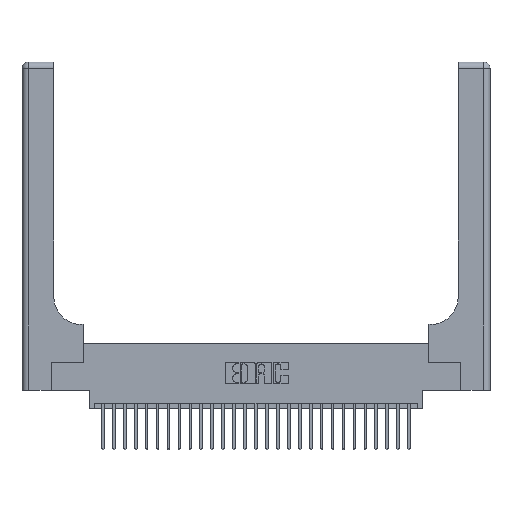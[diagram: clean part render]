
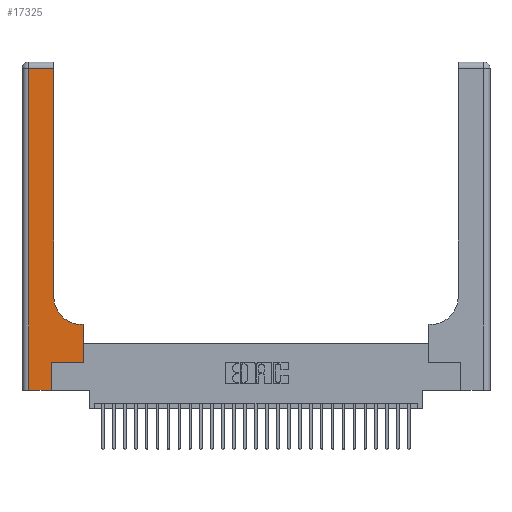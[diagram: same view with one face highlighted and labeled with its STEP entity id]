
A CAD part, top view. The second image highlights one B-rep face of the part: STEP entity #17325.
In plain terms, the highlighted planar face has unit normal (0, 0, 1).
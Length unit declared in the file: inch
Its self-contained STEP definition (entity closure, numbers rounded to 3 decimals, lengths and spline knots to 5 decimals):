
#1298 = LINE ( 'NONE', #27230, #19099 ) ;
#1423 = CARTESIAN_POINT ( 'NONE',  ( 0., 0., 0.37 ) ) ;
#1466 = EDGE_CURVE ( 'NONE', #2934, #4281, #10617, .T. ) ;
#1801 = LINE ( 'NONE', #24195, #18869 ) ;
#2200 = DIRECTION ( 'NONE',  ( 0., 0., -1. ) ) ;
#2375 = CARTESIAN_POINT ( 'NONE',  ( 0.06, 0., 0.37 ) ) ;
#2383 = LINE ( 'NONE', #25163, #8581 ) ;
#2589 = CARTESIAN_POINT ( 'NONE',  ( 0.2915, 0.85, 0.37 ) ) ;
#2788 = ORIENTED_EDGE ( 'NONE', *, *, #9597, .T. ) ;
#2934 = VERTEX_POINT ( 'NONE', #28388 ) ;
#4281 = VERTEX_POINT ( 'NONE', #19247 ) ;
#4468 = DIRECTION ( 'NONE',  ( 0., 1., 0. ) ) ;
#4503 = ORIENTED_EDGE ( 'NONE', *, *, #10538, .T. ) ;
#5629 = ORIENTED_EDGE ( 'NONE', *, *, #15388, .T. ) ;
#5668 = DIRECTION ( 'NONE',  ( 0., -1., 0. ) ) ;
#6126 = VECTOR ( 'NONE', #29009, 39.37008 ) ;
#6192 = CARTESIAN_POINT ( 'NONE',  ( 0.06, 3., 0.37 ) ) ;
#7147 = VERTEX_POINT ( 'NONE', #21695 ) ;
#7614 = ORIENTED_EDGE ( 'NONE', *, *, #24966, .T. ) ;
#8573 = ORIENTED_EDGE ( 'NONE', *, *, #11601, .T. ) ;
#8581 = VECTOR ( 'NONE', #8957, 39.37008 ) ;
#8632 = AXIS2_PLACEMENT_3D ( 'NONE', #16107, #2200, #18460 ) ;
#8703 = CARTESIAN_POINT ( 'NONE',  ( 0.269, 0., 0.37 ) ) ;
#8957 = DIRECTION ( 'NONE',  ( 0., 1., 0. ) ) ;
#9030 = CARTESIAN_POINT ( 'NONE',  ( 0.5585, 0.25, 0.37 ) ) ;
#9222 = VERTEX_POINT ( 'NONE', #16015 ) ;
#9597 = EDGE_CURVE ( 'NONE', #4281, #28077, #13017, .T. ) ;
#10387 = CARTESIAN_POINT ( 'NONE',  ( 0.269, 0.25, 0.37 ) ) ;
#10538 = EDGE_CURVE ( 'NONE', #27369, #9222, #2383, .T. ) ;
#10617 = LINE ( 'NONE', #9030, #22215 ) ;
#11234 = CARTESIAN_POINT ( 'NONE',  ( 0., 3., 0.37 ) ) ;
#11256 = EDGE_CURVE ( 'NONE', #28077, #27369, #25201, .T. ) ;
#11601 = EDGE_CURVE ( 'NONE', #17575, #12013, #23376, .T. ) ;
#12013 = VERTEX_POINT ( 'NONE', #2375 ) ;
#12656 = DIRECTION ( 'NONE',  ( 1., 0., 0. ) ) ;
#13004 = EDGE_CURVE ( 'NONE', #12013, #7147, #28109, .T. ) ;
#13017 = LINE ( 'NONE', #22186, #6126 ) ;
#13105 = DIRECTION ( 'NONE',  ( 1., 0., 0. ) ) ;
#13462 = ORIENTED_EDGE ( 'NONE', *, *, #11256, .T. ) ;
#13506 = CARTESIAN_POINT ( 'NONE',  ( 0.06, 2.94, 0.37 ) ) ;
#13559 = DIRECTION ( 'NONE',  ( 0., 0., -1. ) ) ;
#14509 = ORIENTED_EDGE ( 'NONE', *, *, #29144, .T. ) ;
#15388 = EDGE_CURVE ( 'NONE', #7147, #29729, #26289, .T. ) ;
#15989 = VECTOR ( 'NONE', #5668, 39.37008 ) ;
#16015 = CARTESIAN_POINT ( 'NONE',  ( 0.2915, 2.94, 0.37 ) ) ;
#16107 = CARTESIAN_POINT ( 'NONE',  ( 0.5415, 0.85, 0.37 ) ) ;
#17325 = ADVANCED_FACE ( 'NONE', ( #20061 ), #27339, .F. ) ;
#17575 = VERTEX_POINT ( 'NONE', #13506 ) ;
#18460 = DIRECTION ( 'NONE',  ( 1., 0., 0. ) ) ;
#18869 = VECTOR ( 'NONE', #12656, 39.37008 ) ;
#19099 = VECTOR ( 'NONE', #20425, 39.37008 ) ;
#19247 = CARTESIAN_POINT ( 'NONE',  ( 0.5585, 0.6, 0.37 ) ) ;
#19838 = EDGE_LOOP ( 'NONE', ( #4503, #7614, #8573, #25747, #5629, #14509, #27243, #2788, #13462 ) ) ;
#20061 = FACE_OUTER_BOUND ( 'NONE', #19838, .T. ) ;
#20425 = DIRECTION ( 'NONE',  ( -1., 0., 0. ) ) ;
#21695 = CARTESIAN_POINT ( 'NONE',  ( 0.269, 0., 0.37 ) ) ;
#22072 = VECTOR ( 'NONE', #13105, 39.37008 ) ;
#22186 = CARTESIAN_POINT ( 'NONE',  ( 0.2915, 0.6, 0.37 ) ) ;
#22215 = VECTOR ( 'NONE', #4468, 39.37008 ) ;
#23376 = LINE ( 'NONE', #6192, #15989 ) ;
#24195 = CARTESIAN_POINT ( 'NONE',  ( 0.269, 0.25, 0.37 ) ) ;
#24919 = DIRECTION ( 'NONE',  ( 0., 1., 0. ) ) ;
#24966 = EDGE_CURVE ( 'NONE', #9222, #17575, #1298, .T. ) ;
#25163 = CARTESIAN_POINT ( 'NONE',  ( 0.2915, 3., 0.37 ) ) ;
#25201 = CIRCLE ( 'NONE', #8632, 0.25 ) ;
#25747 = ORIENTED_EDGE ( 'NONE', *, *, #13004, .T. ) ;
#26289 = LINE ( 'NONE', #8703, #26979 ) ;
#26979 = VECTOR ( 'NONE', #24919, 39.37008 ) ;
#27230 = CARTESIAN_POINT ( 'NONE',  ( 0., 2.94, 0.37 ) ) ;
#27243 = ORIENTED_EDGE ( 'NONE', *, *, #1466, .T. ) ;
#27339 = PLANE ( 'NONE',  #28416 ) ;
#27369 = VERTEX_POINT ( 'NONE', #2589 ) ;
#28077 = VERTEX_POINT ( 'NONE', #28093 ) ;
#28093 = CARTESIAN_POINT ( 'NONE',  ( 0.5415, 0.6, 0.37 ) ) ;
#28109 = LINE ( 'NONE', #1423, #22072 ) ;
#28388 = CARTESIAN_POINT ( 'NONE',  ( 0.5585, 0.25, 0.37 ) ) ;
#28416 = AXIS2_PLACEMENT_3D ( 'NONE', #11234, #13559, #29593 ) ;
#29009 = DIRECTION ( 'NONE',  ( -1., 0., 0. ) ) ;
#29144 = EDGE_CURVE ( 'NONE', #29729, #2934, #1801, .T. ) ;
#29593 = DIRECTION ( 'NONE',  ( -1., 0., 0. ) ) ;
#29729 = VERTEX_POINT ( 'NONE', #10387 ) ;
